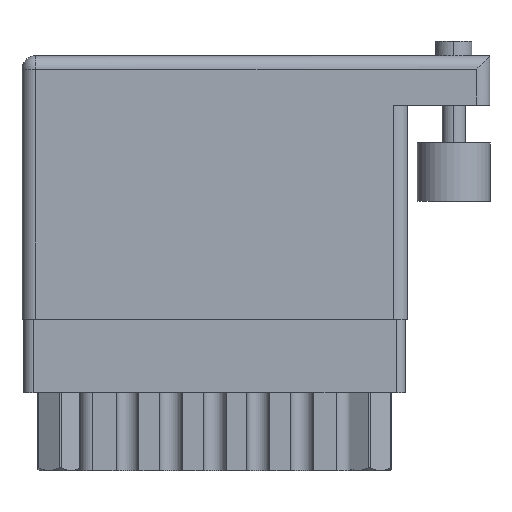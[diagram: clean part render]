
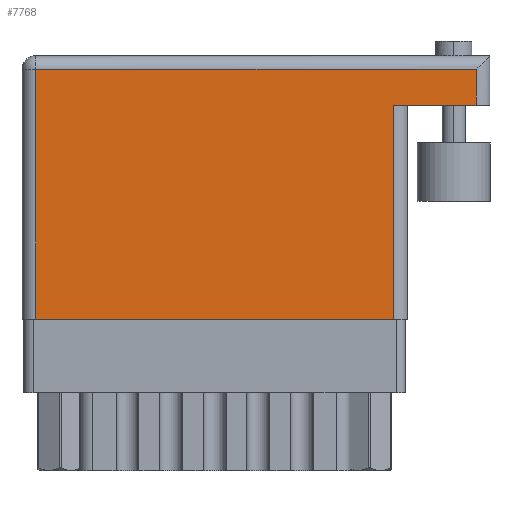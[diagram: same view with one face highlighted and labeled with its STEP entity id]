
A CAD part, front view. The second image highlights one B-rep face of the part: STEP entity #7768.
In plain terms, the highlighted face is planar.
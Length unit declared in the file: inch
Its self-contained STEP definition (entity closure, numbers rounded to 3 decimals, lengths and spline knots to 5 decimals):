
#201 = CARTESIAN_POINT ( 'NONE',  ( 1.562, 0.736, 0. ) ) ;
#903 = EDGE_CURVE ( 'NONE', #4998, #31515, #5569, .T. ) ;
#2487 = VECTOR ( 'NONE', #23890, 39.37008 ) ;
#2862 = DIRECTION ( 'NONE',  ( -1., 0., 0. ) ) ;
#4923 = EDGE_CURVE ( 'NONE', #25606, #9686, #12145, .T. ) ;
#4998 = VERTEX_POINT ( 'NONE', #34334 ) ;
#5345 = CARTESIAN_POINT ( 'NONE',  ( 1.562, 0.906, 0. ) ) ;
#5569 = LINE ( 'NONE', #13447, #11480 ) ;
#5685 = EDGE_CURVE ( 'NONE', #13950, #31515, #32532, .T. ) ;
#6401 = VECTOR ( 'NONE', #24489, 39.37008 ) ;
#7768 = ADVANCED_FACE ( 'NONE', ( #13891 ), #22111, .F. ) ;
#8184 = CARTESIAN_POINT ( 'NONE',  ( 1.278, 0.736, 0. ) ) ;
#8883 = DIRECTION ( 'NONE',  ( 1., 0., 0. ) ) ;
#9686 = VERTEX_POINT ( 'NONE', #11599 ) ;
#10329 = AXIS2_PLACEMENT_3D ( 'NONE', #24732, #24565, #2862 ) ;
#11480 = VECTOR ( 'NONE', #24105, 39.37008 ) ;
#11500 = CARTESIAN_POINT ( 'NONE',  ( 0., 0., 0. ) ) ;
#11599 = CARTESIAN_POINT ( 'NONE',  ( 0.047, 0.859, 0. ) ) ;
#12145 = LINE ( 'NONE', #27893, #27578 ) ;
#12312 = ORIENTED_EDGE ( 'NONE', *, *, #18732, .T. ) ;
#12416 = EDGE_LOOP ( 'NONE', ( #22861, #31471, #15671, #15357, #32863, #12312 ) ) ;
#13447 = CARTESIAN_POINT ( 'NONE',  ( 1.278, 0.736, 0. ) ) ;
#13891 = FACE_OUTER_BOUND ( 'NONE', #12416, .T. ) ;
#13950 = VERTEX_POINT ( 'NONE', #201 ) ;
#14146 = CARTESIAN_POINT ( 'NONE',  ( 1.609, 0.736, 0. ) ) ;
#14233 = DIRECTION ( 'NONE',  ( -1., 0., 0. ) ) ;
#14764 = EDGE_CURVE ( 'NONE', #13950, #25606, #26700, .T. ) ;
#14840 = VECTOR ( 'NONE', #20445, 39.37008 ) ;
#15357 = ORIENTED_EDGE ( 'NONE', *, *, #14764, .T. ) ;
#15671 = ORIENTED_EDGE ( 'NONE', *, *, #5685, .F. ) ;
#18732 = EDGE_CURVE ( 'NONE', #9686, #30690, #33574, .T. ) ;
#20445 = DIRECTION ( 'NONE',  ( 0., -1., 0. ) ) ;
#21154 = VECTOR ( 'NONE', #8883, 39.37008 ) ;
#22111 = PLANE ( 'NONE',  #10329 ) ;
#22861 = ORIENTED_EDGE ( 'NONE', *, *, #29600, .T. ) ;
#23890 = DIRECTION ( 'NONE',  ( 0., 1., 0. ) ) ;
#24105 = DIRECTION ( 'NONE',  ( 0., 1., 0. ) ) ;
#24489 = DIRECTION ( 'NONE',  ( -1., 0., 0. ) ) ;
#24565 = DIRECTION ( 'NONE',  ( 0., 0., -1. ) ) ;
#24732 = CARTESIAN_POINT ( 'NONE',  ( 0., 0.906, 0. ) ) ;
#25521 = CARTESIAN_POINT ( 'NONE',  ( 0.047, 0., 0. ) ) ;
#25606 = VERTEX_POINT ( 'NONE', #33312 ) ;
#26700 = LINE ( 'NONE', #5345, #2487 ) ;
#27578 = VECTOR ( 'NONE', #14233, 39.37008 ) ;
#27893 = CARTESIAN_POINT ( 'NONE',  ( 0., 0.859, 0. ) ) ;
#29600 = EDGE_CURVE ( 'NONE', #30690, #4998, #30377, .T. ) ;
#30377 = LINE ( 'NONE', #11500, #21154 ) ;
#30690 = VERTEX_POINT ( 'NONE', #31264 ) ;
#31264 = CARTESIAN_POINT ( 'NONE',  ( 0.047, 0., 0. ) ) ;
#31471 = ORIENTED_EDGE ( 'NONE', *, *, #903, .T. ) ;
#31515 = VERTEX_POINT ( 'NONE', #8184 ) ;
#32532 = LINE ( 'NONE', #14146, #6401 ) ;
#32863 = ORIENTED_EDGE ( 'NONE', *, *, #4923, .T. ) ;
#33312 = CARTESIAN_POINT ( 'NONE',  ( 1.562, 0.859, 0. ) ) ;
#33574 = LINE ( 'NONE', #25521, #14840 ) ;
#34334 = CARTESIAN_POINT ( 'NONE',  ( 1.278, 0., 0. ) ) ;
